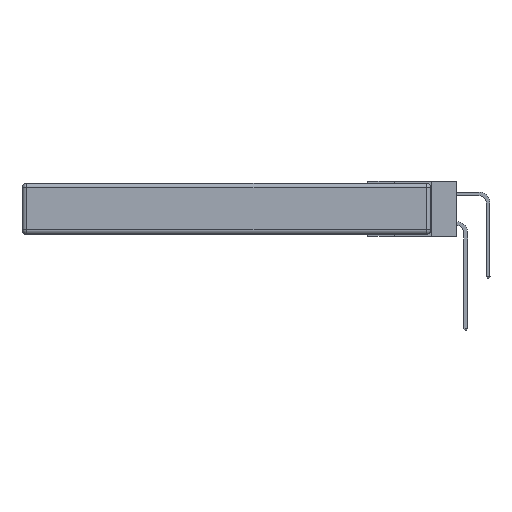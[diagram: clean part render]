
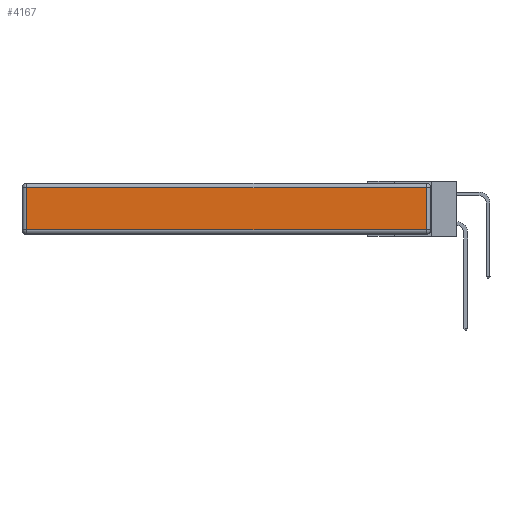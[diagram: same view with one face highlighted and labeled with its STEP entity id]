
A CAD part, left-side view. The second image highlights one B-rep face of the part: STEP entity #4167.
In plain terms, the highlighted planar face has unit normal (-1, 0, 0).
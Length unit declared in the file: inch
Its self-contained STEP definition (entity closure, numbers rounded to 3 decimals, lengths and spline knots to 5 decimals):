
#386 = ORIENTED_EDGE ( 'NONE', *, *, #15350, .T. ) ;
#1759 = AXIS2_PLACEMENT_3D ( 'NONE', #7925, #21417, #15444 ) ;
#2415 = DIRECTION ( 'NONE',  ( 0., 1., 0. ) ) ;
#3786 = EDGE_CURVE ( 'NONE', #22321, #21869, #24254, .T. ) ;
#4167 = ADVANCED_FACE ( 'NONE', ( #17317 ), #5900, .T. ) ;
#4629 = VECTOR ( 'NONE', #16819, 39.37008 ) ;
#4664 = LINE ( 'NONE', #18400, #14357 ) ;
#5900 = PLANE ( 'NONE',  #1759 ) ;
#6120 = VECTOR ( 'NONE', #17251, 39.37008 ) ;
#7336 = CARTESIAN_POINT ( 'NONE',  ( 0., 0., -0.313 ) ) ;
#7840 = CARTESIAN_POINT ( 'NONE',  ( 0., 2.75, -0.03 ) ) ;
#7925 = CARTESIAN_POINT ( 'NONE',  ( 0., 0., -0.343 ) ) ;
#7988 = LINE ( 'NONE', #7840, #21263 ) ;
#9308 = EDGE_CURVE ( 'NONE', #19002, #22321, #7988, .T. ) ;
#9807 = CARTESIAN_POINT ( 'NONE',  ( 0., 2.72, -0.313 ) ) ;
#10352 = EDGE_CURVE ( 'NONE', #21869, #24126, #17300, .T. ) ;
#11890 = EDGE_LOOP ( 'NONE', ( #20704, #386, #22460, #24730 ) ) ;
#14297 = DIRECTION ( 'NONE',  ( 0., 0., 1. ) ) ;
#14357 = VECTOR ( 'NONE', #14297, 39.37008 ) ;
#14461 = CARTESIAN_POINT ( 'NONE',  ( 0., 2.72, -0.03 ) ) ;
#15350 = EDGE_CURVE ( 'NONE', #24126, #19002, #4664, .T. ) ;
#15444 = DIRECTION ( 'NONE',  ( 0., 0., 1. ) ) ;
#16819 = DIRECTION ( 'NONE',  ( 0., 0., -1. ) ) ;
#17251 = DIRECTION ( 'NONE',  ( 0., -1., 0. ) ) ;
#17300 = LINE ( 'NONE', #7336, #6120 ) ;
#17317 = FACE_OUTER_BOUND ( 'NONE', #11890, .T. ) ;
#18400 = CARTESIAN_POINT ( 'NONE',  ( 0., 0.03, -0.343 ) ) ;
#19002 = VERTEX_POINT ( 'NONE', #23230 ) ;
#20704 = ORIENTED_EDGE ( 'NONE', *, *, #10352, .T. ) ;
#20755 = CARTESIAN_POINT ( 'NONE',  ( 0., 2.72, -0.343 ) ) ;
#21263 = VECTOR ( 'NONE', #2415, 39.37008 ) ;
#21417 = DIRECTION ( 'NONE',  ( -1., 0., 0. ) ) ;
#21869 = VERTEX_POINT ( 'NONE', #9807 ) ;
#22321 = VERTEX_POINT ( 'NONE', #14461 ) ;
#22460 = ORIENTED_EDGE ( 'NONE', *, *, #9308, .T. ) ;
#23230 = CARTESIAN_POINT ( 'NONE',  ( 0., 0.03, -0.03 ) ) ;
#23370 = CARTESIAN_POINT ( 'NONE',  ( 0., 0.03, -0.313 ) ) ;
#24126 = VERTEX_POINT ( 'NONE', #23370 ) ;
#24254 = LINE ( 'NONE', #20755, #4629 ) ;
#24730 = ORIENTED_EDGE ( 'NONE', *, *, #3786, .T. ) ;
